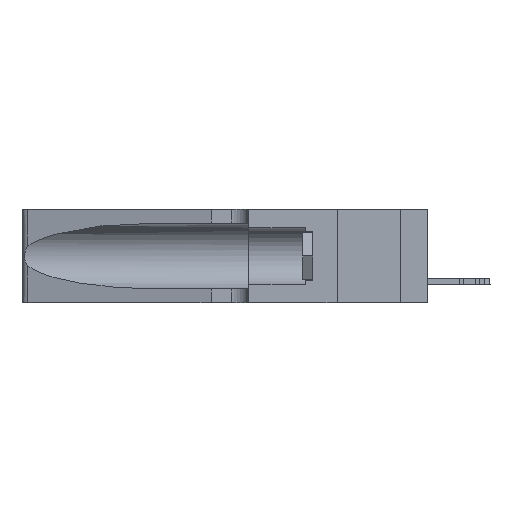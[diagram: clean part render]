
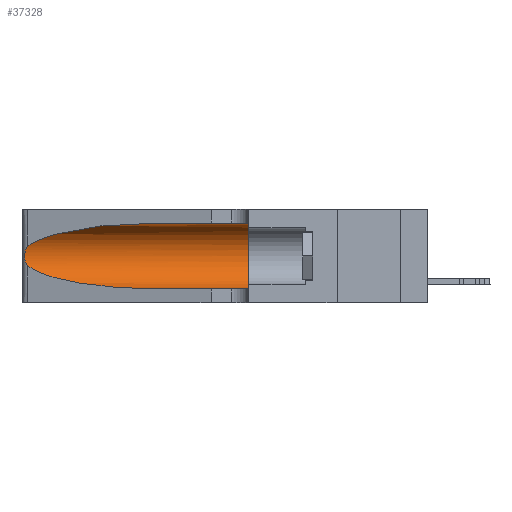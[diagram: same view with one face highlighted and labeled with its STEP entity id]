
A CAD part, left-side view. The second image highlights one B-rep face of the part: STEP entity #37328.
In plain terms, the highlighted cylindrical face has radius 3.308 mm (diameter 6.617 mm), a partial arc.
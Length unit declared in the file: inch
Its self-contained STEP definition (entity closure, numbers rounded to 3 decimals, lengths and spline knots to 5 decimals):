
#306 = AXIS2_PLACEMENT_3D ( 'NONE', #25546, #25734, #18020 ) ;
#1376 = ORIENTED_EDGE ( 'NONE', *, *, #7575, .F. ) ;
#1508 = LINE ( 'NONE', #39436, #31832 ) ;
#1536 = CARTESIAN_POINT ( 'NONE',  ( 0.26018, 1.23835, 0.19895 ) ) ;
#1705 = CARTESIAN_POINT ( 'NONE',  ( 0.25487, 1.22718, 0.22369 ) ) ;
#2356 = DIRECTION ( 'NONE',  ( 0., -1., 0. ) ) ;
#2890 = CARTESIAN_POINT ( 'NONE',  ( 0.25487, 1.22718, 0.14631 ) ) ;
#4433 = EDGE_CURVE ( 'NONE', #28436, #37067, #45207, .T. ) ;
#4476 = ORIENTED_EDGE ( 'NONE', *, *, #24209, .T. ) ;
#5011 = CARTESIAN_POINT ( 'NONE',  ( 0.1305, 0.35, 0.05475 ) ) ;
#5357 = CARTESIAN_POINT ( 'NONE',  ( 0.25856, 1.23593, 0.16098 ) ) ;
#5669 = CARTESIAN_POINT ( 'NONE',  ( 0.1305, 1.61858, 0.31525 ) ) ;
#7575 = EDGE_CURVE ( 'NONE', #17342, #10751, #47752, .T. ) ;
#7638 = EDGE_LOOP ( 'NONE', ( #26643, #28818, #28912, #4476, #15487, #1376 ) ) ;
#10205 = CARTESIAN_POINT ( 'NONE',  ( 0.2373, 1.15595, 0.08982 ) ) ;
#10528 = CARTESIAN_POINT ( 'NONE',  ( 0.1305, 0.72297, 0.05475 ) ) ;
#10751 = VERTEX_POINT ( 'NONE', #20321 ) ;
#12503 = DIRECTION ( 'NONE',  ( 0., -1., 0. ) ) ;
#13029 = CARTESIAN_POINT ( 'NONE',  ( 0.25487, 1.22718, 0.14631 ) ) ;
#14515 = DIRECTION ( 'NONE',  ( 0., 1., 0. ) ) ;
#15487 = ORIENTED_EDGE ( 'NONE', *, *, #35964, .F. ) ;
#16625 = CARTESIAN_POINT ( 'NONE',  ( 0.26017, 1.23833, 0.17102 ) ) ;
#16777 = EDGE_CURVE ( 'NONE', #31735, #28436, #36981, .T. ) ;
#17124 = CARTESIAN_POINT ( 'NONE',  ( 0.25639, 1.23184, 0.21858 ) ) ;
#17342 = VERTEX_POINT ( 'NONE', #30506 ) ;
#17456 = VERTEX_POINT ( 'NONE', #5011 ) ;
#18020 = DIRECTION ( 'NONE',  ( 0., 0., -1. ) ) ;
#20321 = CARTESIAN_POINT ( 'NONE',  ( 0.1305, 0.35, 0.31525 ) ) ;
#20983 = CARTESIAN_POINT ( 'NONE',  ( 0.25555, 1.22994, 0.2215 ) ) ;
#23996 = CARTESIAN_POINT ( 'NONE',  ( 0.1305, 0.72297, 0.05475 ) ) ;
#24133 = AXIS2_PLACEMENT_3D ( 'NONE', #41291, #14515, #41603 ) ;
#24209 = EDGE_CURVE ( 'NONE', #37067, #17456, #1508, .T. ) ;
#25546 = CARTESIAN_POINT ( 'NONE',  ( 0.1305, 1.61858, 0.185 ) ) ;
#25734 = DIRECTION ( 'NONE',  ( 0., -1., 0. ) ) ;
#26018 = CARTESIAN_POINT ( 'NONE',  ( 0.18966, 0.96281, 0.05475 ) ) ;
#26592 =( BOUNDED_CURVE ( )  B_SPLINE_CURVE ( 3, ( #32316, #36198, #47650, #47297 ),
 .UNSPECIFIED., .F., .T. ) 
 B_SPLINE_CURVE_WITH_KNOTS ( ( 4, 4 ),
 ( 1.5708, 2.84003 ),
 .UNSPECIFIED. ) 
 CURVE ( )  GEOMETRIC_REPRESENTATION_ITEM ( )  RATIONAL_B_SPLINE_CURVE ( ( 1., 0.87, 0.87, 1. ) ) 
 REPRESENTATION_ITEM ( '' )  );
#26643 = ORIENTED_EDGE ( 'NONE', *, *, #31418, .T. ) ;
#28114 = VECTOR ( 'NONE', #2356, 39.37008 ) ;
#28162 = CARTESIAN_POINT ( 'NONE',  ( 0.26075, 1.23896, 0.178 ) ) ;
#28436 = VERTEX_POINT ( 'NONE', #31900 ) ;
#28818 = ORIENTED_EDGE ( 'NONE', *, *, #16777, .T. ) ;
#28912 = ORIENTED_EDGE ( 'NONE', *, *, #4433, .T. ) ;
#30506 = CARTESIAN_POINT ( 'NONE',  ( 0.1305, 0.72297, 0.31525 ) ) ;
#31418 = EDGE_CURVE ( 'NONE', #17342, #31735, #26592, .T. ) ;
#31735 = VERTEX_POINT ( 'NONE', #47178 ) ;
#31832 = VECTOR ( 'NONE', #12503, 39.37008 ) ;
#31900 = CARTESIAN_POINT ( 'NONE',  ( 0.25487, 1.22718, 0.14631 ) ) ;
#31934 = CARTESIAN_POINT ( 'NONE',  ( 0.25789, 1.23486, 0.15765 ) ) ;
#32316 = CARTESIAN_POINT ( 'NONE',  ( 0.1305, 0.72297, 0.31525 ) ) ;
#35828 = CARTESIAN_POINT ( 'NONE',  ( 0.25555, 1.22993, 0.14849 ) ) ;
#35964 = EDGE_CURVE ( 'NONE', #10751, #17456, #41296, .T. ) ;
#36198 = CARTESIAN_POINT ( 'NONE',  ( 0.18966, 0.96281, 0.31525 ) ) ;
#36334 = CARTESIAN_POINT ( 'NONE',  ( 0.26075, 1.23896, 0.19203 ) ) ;
#36981 = B_SPLINE_CURVE_WITH_KNOTS ( 'NONE', 3,
 ( #1705, #20983, #17124, #39614, #47798, #1536, #36334, #28162, #16625, #5357, #31934, #47428, #35828, #13029 ),
 .UNSPECIFIED., .F., .F.,
 ( 4, 2, 2, 2, 2, 2, 4 ),
 ( 0., 0.00027, 0.00053, 0.00107, 0.0016, 0.00187, 0.00214 ),
 .UNSPECIFIED. ) ;
#37067 = VERTEX_POINT ( 'NONE', #23996 ) ;
#37328 = ADVANCED_FACE ( 'NONE', ( #43439 ), #44701, .F. ) ;
#39436 = CARTESIAN_POINT ( 'NONE',  ( 0.1305, 1.61858, 0.05475 ) ) ;
#39614 = CARTESIAN_POINT ( 'NONE',  ( 0.25787, 1.23484, 0.2124 ) ) ;
#41291 = CARTESIAN_POINT ( 'NONE',  ( 0.1305, 0.35, 0.185 ) ) ;
#41296 = CIRCLE ( 'NONE', #24133, 0.13025 ) ;
#41603 = DIRECTION ( 'NONE',  ( 0., 0., 1. ) ) ;
#43439 = FACE_OUTER_BOUND ( 'NONE', #7638, .T. ) ;
#44701 = CYLINDRICAL_SURFACE ( 'NONE', #306, 0.13025 ) ;
#45207 =( BOUNDED_CURVE ( )  B_SPLINE_CURVE ( 3, ( #2890, #10205, #26018, #10528 ),
 .UNSPECIFIED., .F., .F. ) 
 B_SPLINE_CURVE_WITH_KNOTS ( ( 4, 4 ),
 ( 3.44316, 4.71239 ),
 .UNSPECIFIED. ) 
 CURVE ( )  GEOMETRIC_REPRESENTATION_ITEM ( )  RATIONAL_B_SPLINE_CURVE ( ( 1., 0.87, 0.87, 1. ) ) 
 REPRESENTATION_ITEM ( '' )  );
#47178 = CARTESIAN_POINT ( 'NONE',  ( 0.25487, 1.22718, 0.22369 ) ) ;
#47297 = CARTESIAN_POINT ( 'NONE',  ( 0.25487, 1.22718, 0.22369 ) ) ;
#47428 = CARTESIAN_POINT ( 'NONE',  ( 0.25639, 1.23186, 0.15144 ) ) ;
#47650 = CARTESIAN_POINT ( 'NONE',  ( 0.2373, 1.15595, 0.28018 ) ) ;
#47752 = LINE ( 'NONE', #5669, #28114 ) ;
#47798 = CARTESIAN_POINT ( 'NONE',  ( 0.25854, 1.2359, 0.20912 ) ) ;
